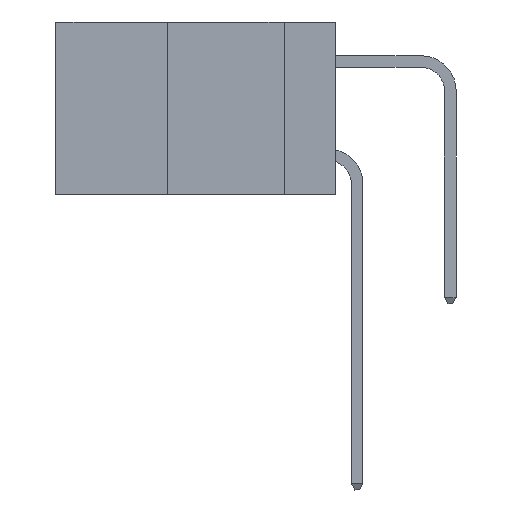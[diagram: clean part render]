
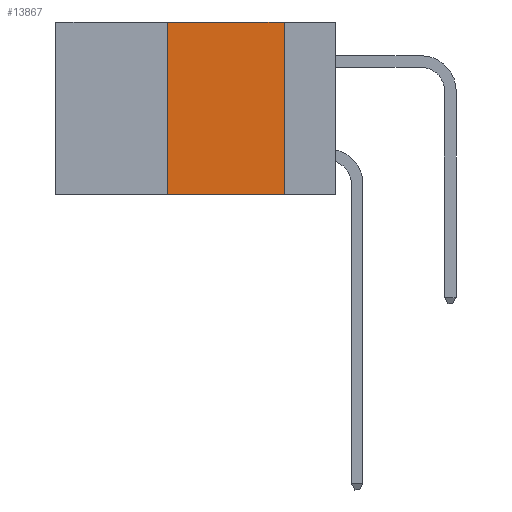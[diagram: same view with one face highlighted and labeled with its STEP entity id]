
A CAD part, left-side view. The second image highlights one B-rep face of the part: STEP entity #13867.
In plain terms, the highlighted planar face has unit normal (-1, 0, 0).
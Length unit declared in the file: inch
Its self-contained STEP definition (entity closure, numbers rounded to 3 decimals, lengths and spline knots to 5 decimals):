
#725 = DIRECTION ( 'NONE',  ( 0., 0., -1. ) ) ;
#1309 = CARTESIAN_POINT ( 'NONE',  ( 0., 0.11, 0. ) ) ;
#1641 = ORIENTED_EDGE ( 'NONE', *, *, #16109, .F. ) ;
#1926 = LINE ( 'NONE', #10565, #23433 ) ;
#2676 = LINE ( 'NONE', #1309, #21591 ) ;
#3238 = EDGE_LOOP ( 'NONE', ( #18054, #12758, #1641, #26720 ) ) ;
#5257 = VERTEX_POINT ( 'NONE', #28111 ) ;
#5416 = CARTESIAN_POINT ( 'NONE',  ( 0., 0.6, 0. ) ) ;
#5867 = DIRECTION ( 'NONE',  ( 0., 0., 1. ) ) ;
#7652 = FACE_OUTER_BOUND ( 'NONE', #3238, .T. ) ;
#9307 = AXIS2_PLACEMENT_3D ( 'NONE', #5416, #12596, #725 ) ;
#10153 = CARTESIAN_POINT ( 'NONE',  ( 0., 0.11, 0. ) ) ;
#10565 = CARTESIAN_POINT ( 'NONE',  ( 0., 0.36, 0. ) ) ;
#10654 = DIRECTION ( 'NONE',  ( 0., -1., 0. ) ) ;
#11417 = VECTOR ( 'NONE', #10654, 39.37008 ) ;
#12596 = DIRECTION ( 'NONE',  ( 1., 0., 0. ) ) ;
#12758 = ORIENTED_EDGE ( 'NONE', *, *, #12972, .F. ) ;
#12804 = LINE ( 'NONE', #24330, #13184 ) ;
#12972 = EDGE_CURVE ( 'NONE', #13046, #26486, #18062, .T. ) ;
#13046 = VERTEX_POINT ( 'NONE', #30039 ) ;
#13184 = VECTOR ( 'NONE', #19602, 39.37008 ) ;
#13867 = ADVANCED_FACE ( 'NONE', ( #7652 ), #19632, .F. ) ;
#14445 = EDGE_CURVE ( 'NONE', #15944, #5257, #12804, .T. ) ;
#14857 = CARTESIAN_POINT ( 'NONE',  ( 0., 0.36, -0.37 ) ) ;
#15944 = VERTEX_POINT ( 'NONE', #14857 ) ;
#16109 = EDGE_CURVE ( 'NONE', #15944, #13046, #1926, .T. ) ;
#16363 = EDGE_CURVE ( 'NONE', #26486, #5257, #2676, .T. ) ;
#17708 = DIRECTION ( 'NONE',  ( 0., 0., -1. ) ) ;
#18054 = ORIENTED_EDGE ( 'NONE', *, *, #16363, .F. ) ;
#18062 = LINE ( 'NONE', #20156, #11417 ) ;
#19602 = DIRECTION ( 'NONE',  ( 0., -1., 0. ) ) ;
#19632 = PLANE ( 'NONE',  #9307 ) ;
#20156 = CARTESIAN_POINT ( 'NONE',  ( 0., 0.6, 0. ) ) ;
#21591 = VECTOR ( 'NONE', #17708, 39.37008 ) ;
#23433 = VECTOR ( 'NONE', #5867, 39.37008 ) ;
#24330 = CARTESIAN_POINT ( 'NONE',  ( 0., 0.6, -0.37 ) ) ;
#26486 = VERTEX_POINT ( 'NONE', #10153 ) ;
#26720 = ORIENTED_EDGE ( 'NONE', *, *, #14445, .T. ) ;
#28111 = CARTESIAN_POINT ( 'NONE',  ( 0., 0.11, -0.37 ) ) ;
#30039 = CARTESIAN_POINT ( 'NONE',  ( 0., 0.36, 0. ) ) ;
